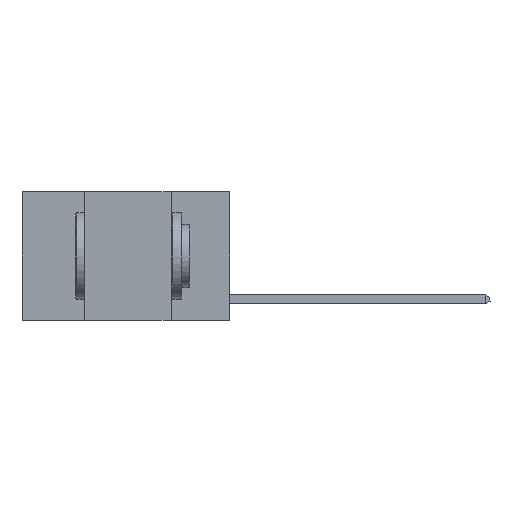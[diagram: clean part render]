
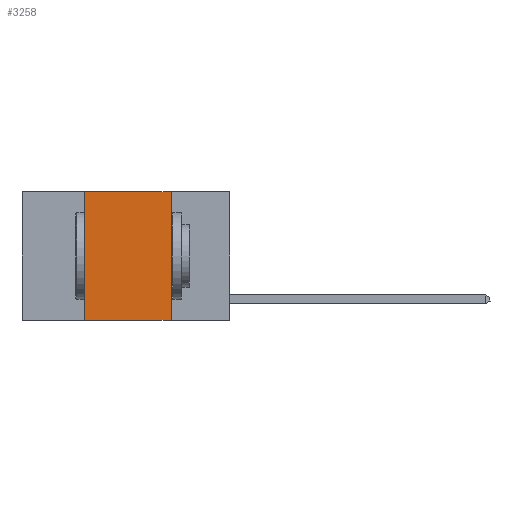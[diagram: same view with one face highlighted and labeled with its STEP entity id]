
A CAD part, left-side view. The second image highlights one B-rep face of the part: STEP entity #3258.
In plain terms, the highlighted planar face has unit normal (-1, 0, 0).
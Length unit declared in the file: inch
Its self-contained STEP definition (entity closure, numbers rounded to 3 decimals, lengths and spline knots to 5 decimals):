
#123 = VECTOR ( 'NONE', #5913, 39.37008 ) ;
#755 = VERTEX_POINT ( 'NONE', #7568 ) ;
#1282 = PLANE ( 'NONE',  #3674 ) ;
#1494 = DIRECTION ( 'NONE',  ( 1., 0., 0. ) ) ;
#2358 = DIRECTION ( 'NONE',  ( 0., 0., -1. ) ) ;
#2910 = EDGE_LOOP ( 'NONE', ( #7187, #12835, #6688, #5397 ) ) ;
#3258 = ADVANCED_FACE ( 'NONE', ( #11006 ), #1282, .F. ) ;
#3502 = EDGE_CURVE ( 'NONE', #8255, #5054, #4173, .T. ) ;
#3674 = AXIS2_PLACEMENT_3D ( 'NONE', #5685, #1494, #2358 ) ;
#3732 = CARTESIAN_POINT ( 'NONE',  ( 0., 0.42, 0. ) ) ;
#4173 = LINE ( 'NONE', #9796, #11423 ) ;
#5054 = VERTEX_POINT ( 'NONE', #3732 ) ;
#5251 = EDGE_CURVE ( 'NONE', #5054, #755, #11838, .T. ) ;
#5397 = ORIENTED_EDGE ( 'NONE', *, *, #10682, .T. ) ;
#5685 = CARTESIAN_POINT ( 'NONE',  ( 0., 0.6, 0. ) ) ;
#5840 = LINE ( 'NONE', #12408, #123 ) ;
#5868 = DIRECTION ( 'NONE',  ( 0., -1., 0. ) ) ;
#5913 = DIRECTION ( 'NONE',  ( 0., 0., -1. ) ) ;
#6688 = ORIENTED_EDGE ( 'NONE', *, *, #3502, .F. ) ;
#7187 = ORIENTED_EDGE ( 'NONE', *, *, #8205, .F. ) ;
#7406 = DIRECTION ( 'NONE',  ( 0., -1., 0. ) ) ;
#7568 = CARTESIAN_POINT ( 'NONE',  ( 0., 0.17, 0. ) ) ;
#8034 = CARTESIAN_POINT ( 'NONE',  ( 0., 0.42, -0.37 ) ) ;
#8205 = EDGE_CURVE ( 'NONE', #755, #11611, #5840, .T. ) ;
#8255 = VERTEX_POINT ( 'NONE', #8034 ) ;
#8853 = VECTOR ( 'NONE', #5868, 39.37008 ) ;
#9463 = VECTOR ( 'NONE', #7406, 39.37008 ) ;
#9796 = CARTESIAN_POINT ( 'NONE',  ( 0., 0.42, 0. ) ) ;
#10129 = LINE ( 'NONE', #13213, #8853 ) ;
#10682 = EDGE_CURVE ( 'NONE', #8255, #11611, #10129, .T. ) ;
#10756 = CARTESIAN_POINT ( 'NONE',  ( 0., 0.17, -0.37 ) ) ;
#11006 = FACE_OUTER_BOUND ( 'NONE', #2910, .T. ) ;
#11423 = VECTOR ( 'NONE', #14011, 39.37008 ) ;
#11611 = VERTEX_POINT ( 'NONE', #10756 ) ;
#11838 = LINE ( 'NONE', #13934, #9463 ) ;
#12408 = CARTESIAN_POINT ( 'NONE',  ( 0., 0.17, 0. ) ) ;
#12835 = ORIENTED_EDGE ( 'NONE', *, *, #5251, .F. ) ;
#13213 = CARTESIAN_POINT ( 'NONE',  ( 0., 0.6, -0.37 ) ) ;
#13934 = CARTESIAN_POINT ( 'NONE',  ( 0., 0.6, 0. ) ) ;
#14011 = DIRECTION ( 'NONE',  ( 0., 0., 1. ) ) ;
